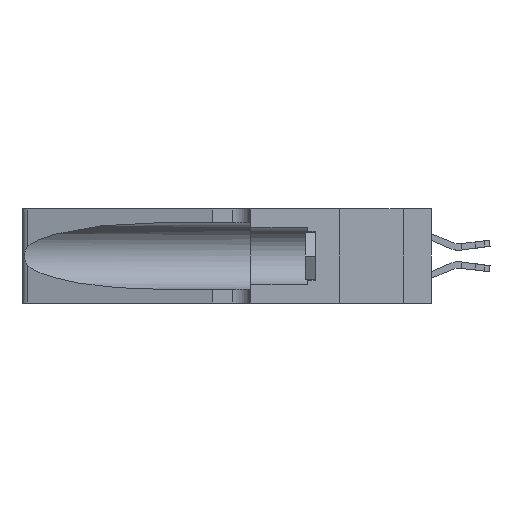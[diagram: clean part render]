
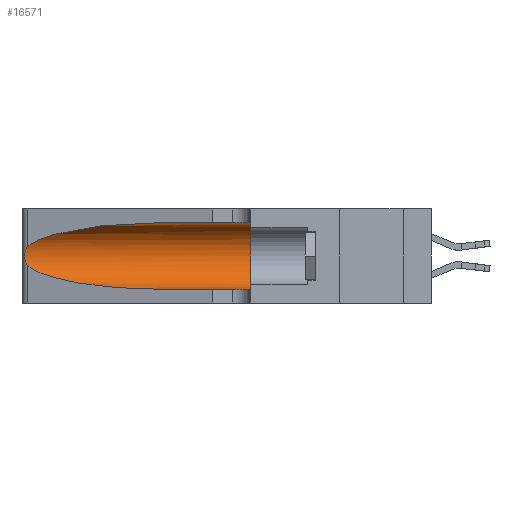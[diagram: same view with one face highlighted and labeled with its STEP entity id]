
A CAD part, left-side view. The second image highlights one B-rep face of the part: STEP entity #16571.
In plain terms, the highlighted cylindrical face has radius 3.308 mm (diameter 6.617 mm), a partial arc.
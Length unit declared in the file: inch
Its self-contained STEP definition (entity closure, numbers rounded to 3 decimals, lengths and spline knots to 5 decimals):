
#162 = CARTESIAN_POINT ( 'NONE',  ( 0.26017, 1.23833, 0.17102 ) ) ;
#490 = CARTESIAN_POINT ( 'NONE',  ( 0.25487, 1.22718, 0.22369 ) ) ;
#1303 = CARTESIAN_POINT ( 'NONE',  ( 0.26075, 1.23896, 0.19203 ) ) ;
#1638 = EDGE_CURVE ( 'NONE', #8650, #14446, #19011, .T. ) ;
#1705 = EDGE_LOOP ( 'NONE', ( #16892, #15435, #4551, #24946, #24598, #27948 ) ) ;
#2585 = CARTESIAN_POINT ( 'NONE',  ( 0.26075, 1.23896, 0.178 ) ) ;
#2603 = EDGE_CURVE ( 'NONE', #3881, #16948, #3016, .T. ) ;
#3016 = LINE ( 'NONE', #28022, #21021 ) ;
#3881 = VERTEX_POINT ( 'NONE', #16534 ) ;
#4015 = CARTESIAN_POINT ( 'NONE',  ( 0.26018, 1.23835, 0.19895 ) ) ;
#4551 = ORIENTED_EDGE ( 'NONE', *, *, #18306, .T. ) ;
#5316 = CARTESIAN_POINT ( 'NONE',  ( 0.25856, 1.23593, 0.16098 ) ) ;
#6210 = DIRECTION ( 'NONE',  ( 0., -1., 0. ) ) ;
#6912 = CARTESIAN_POINT ( 'NONE',  ( 0.1305, 1.61858, 0.185 ) ) ;
#7354 = CARTESIAN_POINT ( 'NONE',  ( 0.18966, 0.96281, 0.31525 ) ) ;
#7586 = CARTESIAN_POINT ( 'NONE',  ( 0.25487, 1.22718, 0.14631 ) ) ;
#7787 = CARTESIAN_POINT ( 'NONE',  ( 0.25555, 1.22993, 0.14849 ) ) ;
#8650 = VERTEX_POINT ( 'NONE', #12287 ) ;
#9823 = VERTEX_POINT ( 'NONE', #25469 ) ;
#9852 = CARTESIAN_POINT ( 'NONE',  ( 0.25487, 1.22718, 0.14631 ) ) ;
#9880 = CARTESIAN_POINT ( 'NONE',  ( 0.1305, 0.72297, 0.31525 ) ) ;
#9981 = AXIS2_PLACEMENT_3D ( 'NONE', #25178, #11819, #27373 ) ;
#10406 = EDGE_CURVE ( 'NONE', #22178, #8650, #16857, .T. ) ;
#10469 = CARTESIAN_POINT ( 'NONE',  ( 0.1305, 0.35, 0.05475 ) ) ;
#10483 = CARTESIAN_POINT ( 'NONE',  ( 0.25787, 1.23484, 0.2124 ) ) ;
#11051 = FACE_OUTER_BOUND ( 'NONE', #1705, .T. ) ;
#11373 = CARTESIAN_POINT ( 'NONE',  ( 0.25639, 1.23184, 0.21858 ) ) ;
#11395 = EDGE_CURVE ( 'NONE', #22178, #9823, #16248, .T. ) ;
#11467 = CARTESIAN_POINT ( 'NONE',  ( 0.25854, 1.2359, 0.20912 ) ) ;
#11819 = DIRECTION ( 'NONE',  ( 0., 1., 0. ) ) ;
#11833 = EDGE_CURVE ( 'NONE', #9823, #16948, #23180, .T. ) ;
#12128 = CARTESIAN_POINT ( 'NONE',  ( 0.18966, 0.96281, 0.05475 ) ) ;
#12287 = CARTESIAN_POINT ( 'NONE',  ( 0.25487, 1.22718, 0.22369 ) ) ;
#12843 = CARTESIAN_POINT ( 'NONE',  ( 0.25639, 1.23186, 0.15144 ) ) ;
#14181 = CARTESIAN_POINT ( 'NONE',  ( 0.2373, 1.15595, 0.28018 ) ) ;
#14446 = VERTEX_POINT ( 'NONE', #17845 ) ;
#14765 = DIRECTION ( 'NONE',  ( 0., -1., 0. ) ) ;
#14867 = VECTOR ( 'NONE', #6210, 39.37008 ) ;
#15435 = ORIENTED_EDGE ( 'NONE', *, *, #1638, .T. ) ;
#15852 = CARTESIAN_POINT ( 'NONE',  ( 0.25789, 1.23486, 0.15765 ) ) ;
#16248 = LINE ( 'NONE', #19678, #14867 ) ;
#16534 = CARTESIAN_POINT ( 'NONE',  ( 0.1305, 0.72297, 0.05475 ) ) ;
#16571 = ADVANCED_FACE ( 'NONE', ( #11051 ), #28086, .F. ) ;
#16857 =( BOUNDED_CURVE ( )  B_SPLINE_CURVE ( 3, ( #22942, #7354, #14181, #490 ),
 .UNSPECIFIED., .F., .F. ) 
 B_SPLINE_CURVE_WITH_KNOTS ( ( 4, 4 ),
 ( 1.5708, 2.84003 ),
 .UNSPECIFIED. ) 
 CURVE ( )  GEOMETRIC_REPRESENTATION_ITEM ( )  RATIONAL_B_SPLINE_CURVE ( ( 1., 0.87, 0.87, 1. ) ) 
 REPRESENTATION_ITEM ( '' )  );
#16892 = ORIENTED_EDGE ( 'NONE', *, *, #10406, .T. ) ;
#16948 = VERTEX_POINT ( 'NONE', #10469 ) ;
#17845 = CARTESIAN_POINT ( 'NONE',  ( 0.25487, 1.22718, 0.14631 ) ) ;
#18122 = DIRECTION ( 'NONE',  ( 0., -1., 0. ) ) ;
#18306 = EDGE_CURVE ( 'NONE', #14446, #3881, #25074, .T. ) ;
#18780 = CARTESIAN_POINT ( 'NONE',  ( 0.2373, 1.15595, 0.08982 ) ) ;
#19011 = B_SPLINE_CURVE_WITH_KNOTS ( 'NONE', 3,
 ( #24104, #22578, #11373, #10483, #11467, #4015, #1303, #2585, #162, #5316, #15852, #12843, #7787, #9852 ),
 .UNSPECIFIED., .F., .F.,
 ( 4, 2, 2, 2, 2, 2, 4 ),
 ( 0., 0.00027, 0.00053, 0.00107, 0.0016, 0.00187, 0.00214 ),
 .UNSPECIFIED. ) ;
#19678 = CARTESIAN_POINT ( 'NONE',  ( 0.1305, 1.61858, 0.31525 ) ) ;
#20180 = DIRECTION ( 'NONE',  ( 0., 0., -1. ) ) ;
#21021 = VECTOR ( 'NONE', #14765, 39.37008 ) ;
#22178 = VERTEX_POINT ( 'NONE', #9880 ) ;
#22578 = CARTESIAN_POINT ( 'NONE',  ( 0.25555, 1.22994, 0.2215 ) ) ;
#22942 = CARTESIAN_POINT ( 'NONE',  ( 0.1305, 0.72297, 0.31525 ) ) ;
#23180 = CIRCLE ( 'NONE', #9981, 0.13025 ) ;
#24104 = CARTESIAN_POINT ( 'NONE',  ( 0.25487, 1.22718, 0.22369 ) ) ;
#24598 = ORIENTED_EDGE ( 'NONE', *, *, #11833, .F. ) ;
#24641 = AXIS2_PLACEMENT_3D ( 'NONE', #6912, #18122, #20180 ) ;
#24946 = ORIENTED_EDGE ( 'NONE', *, *, #2603, .T. ) ;
#25074 =( BOUNDED_CURVE ( )  B_SPLINE_CURVE ( 3, ( #7586, #18780, #12128, #27663 ),
 .UNSPECIFIED., .F., .F. ) 
 B_SPLINE_CURVE_WITH_KNOTS ( ( 4, 4 ),
 ( 3.44316, 4.71239 ),
 .UNSPECIFIED. ) 
 CURVE ( )  GEOMETRIC_REPRESENTATION_ITEM ( )  RATIONAL_B_SPLINE_CURVE ( ( 1., 0.87, 0.87, 1. ) ) 
 REPRESENTATION_ITEM ( '' )  );
#25178 = CARTESIAN_POINT ( 'NONE',  ( 0.1305, 0.35, 0.185 ) ) ;
#25469 = CARTESIAN_POINT ( 'NONE',  ( 0.1305, 0.35, 0.31525 ) ) ;
#27373 = DIRECTION ( 'NONE',  ( 0., 0., 1. ) ) ;
#27663 = CARTESIAN_POINT ( 'NONE',  ( 0.1305, 0.72297, 0.05475 ) ) ;
#27948 = ORIENTED_EDGE ( 'NONE', *, *, #11395, .F. ) ;
#28022 = CARTESIAN_POINT ( 'NONE',  ( 0.1305, 1.61858, 0.05475 ) ) ;
#28086 = CYLINDRICAL_SURFACE ( 'NONE', #24641, 0.13025 ) ;
